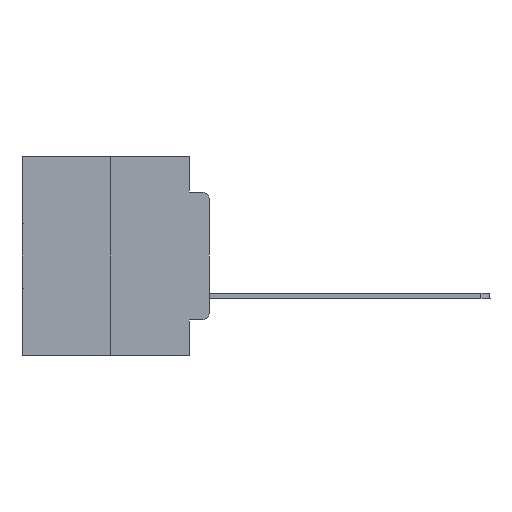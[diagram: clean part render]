
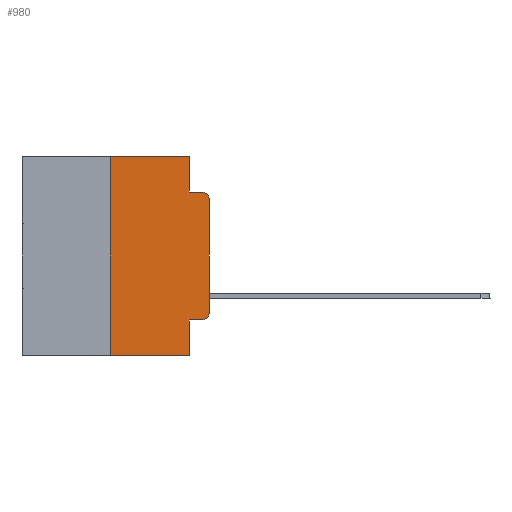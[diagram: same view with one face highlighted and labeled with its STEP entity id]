
A CAD part, left-side view. The second image highlights one B-rep face of the part: STEP entity #980.
In plain terms, the highlighted planar face has unit normal (-1, 0, 0).
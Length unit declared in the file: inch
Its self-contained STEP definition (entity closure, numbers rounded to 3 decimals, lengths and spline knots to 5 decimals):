
#5 = VECTOR ( 'NONE', #29559, 39.37008 ) ;
#486 = CARTESIAN_POINT ( 'NONE',  ( 0., 0., -0.3915 ) ) ;
#980 = ADVANCED_FACE ( 'NONE', ( #6678 ), #12092, .F. ) ;
#1792 = AXIS2_PLACEMENT_3D ( 'NONE', #6769, #27558, #7856 ) ;
#2124 = DIRECTION ( 'NONE',  ( 0., 0., -1. ) ) ;
#2141 = CARTESIAN_POINT ( 'NONE',  ( 0., 0.02, -0.1085 ) ) ;
#2211 = VERTEX_POINT ( 'NONE', #11360 ) ;
#2654 = VERTEX_POINT ( 'NONE', #27914 ) ;
#3202 = VERTEX_POINT ( 'NONE', #486 ) ;
#3818 = CARTESIAN_POINT ( 'NONE',  ( 0., 0.02, -0.0885 ) ) ;
#4131 = EDGE_CURVE ( 'NONE', #4163, #14780, #28726, .T. ) ;
#4163 = VERTEX_POINT ( 'NONE', #23117 ) ;
#4250 = EDGE_CURVE ( 'NONE', #11388, #4163, #6954, .T. ) ;
#4488 = DIRECTION ( 'NONE',  ( 0., -1., 0. ) ) ;
#4757 = VERTEX_POINT ( 'NONE', #7242 ) ;
#4994 = ORIENTED_EDGE ( 'NONE', *, *, #28750, .T. ) ;
#5087 = LINE ( 'NONE', #17276, #20365 ) ;
#5193 = ORIENTED_EDGE ( 'NONE', *, *, #13440, .F. ) ;
#5793 = EDGE_LOOP ( 'NONE', ( #4994, #28926, #23250, #27149, #14886, #5193, #23694, #9045, #26139, #23555 ) ) ;
#6230 = VERTEX_POINT ( 'NONE', #18127 ) ;
#6678 = FACE_OUTER_BOUND ( 'NONE', #5793, .T. ) ;
#6769 = CARTESIAN_POINT ( 'NONE',  ( 0., 0.02, -0.3915 ) ) ;
#6954 = LINE ( 'NONE', #18307, #26534 ) ;
#6980 = LINE ( 'NONE', #30104, #10633 ) ;
#7242 = CARTESIAN_POINT ( 'NONE',  ( 0., 0.02, -0.4115 ) ) ;
#7600 = DIRECTION ( 'NONE',  ( 1., 0., 0. ) ) ;
#7856 = DIRECTION ( 'NONE',  ( 0., 0., -1. ) ) ;
#7988 = LINE ( 'NONE', #10809, #5 ) ;
#8258 = EDGE_CURVE ( 'NONE', #4757, #3202, #11803, .T. ) ;
#9045 = ORIENTED_EDGE ( 'NONE', *, *, #11164, .F. ) ;
#10145 = DIRECTION ( 'NONE',  ( 0., 0., 1. ) ) ;
#10633 = VECTOR ( 'NONE', #22979, 39.37008 ) ;
#10809 = CARTESIAN_POINT ( 'NONE',  ( 0., 0.473, -0.5 ) ) ;
#10830 = CARTESIAN_POINT ( 'NONE',  ( 0., 0.25, 0. ) ) ;
#11164 = EDGE_CURVE ( 'NONE', #6230, #27643, #5087, .T. ) ;
#11336 = CIRCLE ( 'NONE', #18917, 0.02 ) ;
#11360 = CARTESIAN_POINT ( 'NONE',  ( 0., 0., -0.1085 ) ) ;
#11376 = DIRECTION ( 'NONE',  ( -1., 0., 0. ) ) ;
#11388 = VERTEX_POINT ( 'NONE', #22035 ) ;
#11675 = CARTESIAN_POINT ( 'NONE',  ( 0., 0.473, 0. ) ) ;
#11803 = CIRCLE ( 'NONE', #1792, 0.02 ) ;
#12092 = PLANE ( 'NONE',  #18562 ) ;
#12635 = EDGE_CURVE ( 'NONE', #6230, #4757, #17356, .T. ) ;
#12959 = DIRECTION ( 'NONE',  ( 0., -1., 0. ) ) ;
#13440 = EDGE_CURVE ( 'NONE', #2654, #28687, #27146, .T. ) ;
#14780 = VERTEX_POINT ( 'NONE', #3818 ) ;
#14886 = ORIENTED_EDGE ( 'NONE', *, *, #25388, .F. ) ;
#15371 = VECTOR ( 'NONE', #27470, 39.37008 ) ;
#15845 = CARTESIAN_POINT ( 'NONE',  ( 0., 0.051, -0.5 ) ) ;
#15999 = VECTOR ( 'NONE', #4488, 39.37008 ) ;
#16795 = CARTESIAN_POINT ( 'NONE',  ( 0., 0.473, 0. ) ) ;
#17162 = LINE ( 'NONE', #11675, #15371 ) ;
#17204 = CARTESIAN_POINT ( 'NONE',  ( 0., 0.25, 0. ) ) ;
#17276 = CARTESIAN_POINT ( 'NONE',  ( 0., 0.051, 0. ) ) ;
#17356 = LINE ( 'NONE', #27159, #22090 ) ;
#18127 = CARTESIAN_POINT ( 'NONE',  ( 0., 0.051, -0.4115 ) ) ;
#18307 = CARTESIAN_POINT ( 'NONE',  ( 0., 0.051, 0. ) ) ;
#18562 = AXIS2_PLACEMENT_3D ( 'NONE', #16795, #7600, #23817 ) ;
#18917 = AXIS2_PLACEMENT_3D ( 'NONE', #2141, #11376, #27559 ) ;
#19114 = DIRECTION ( 'NONE',  ( 0., 0., -1. ) ) ;
#20365 = VECTOR ( 'NONE', #19114, 39.37008 ) ;
#21574 = EDGE_CURVE ( 'NONE', #2211, #14780, #11336, .T. ) ;
#22035 = CARTESIAN_POINT ( 'NONE',  ( 0., 0.051, 0. ) ) ;
#22090 = VECTOR ( 'NONE', #12959, 39.37008 ) ;
#22979 = DIRECTION ( 'NONE',  ( 0., 0., 1. ) ) ;
#23117 = CARTESIAN_POINT ( 'NONE',  ( 0., 0.051, -0.0885 ) ) ;
#23250 = ORIENTED_EDGE ( 'NONE', *, *, #4131, .F. ) ;
#23555 = ORIENTED_EDGE ( 'NONE', *, *, #8258, .T. ) ;
#23694 = ORIENTED_EDGE ( 'NONE', *, *, #29824, .T. ) ;
#23817 = DIRECTION ( 'NONE',  ( 0., 0., -1. ) ) ;
#24615 = VECTOR ( 'NONE', #10145, 39.37008 ) ;
#25174 = CARTESIAN_POINT ( 'NONE',  ( 0., 0.051, -0.0885 ) ) ;
#25388 = EDGE_CURVE ( 'NONE', #28687, #11388, #17162, .T. ) ;
#26139 = ORIENTED_EDGE ( 'NONE', *, *, #12635, .T. ) ;
#26534 = VECTOR ( 'NONE', #2124, 39.37008 ) ;
#27146 = LINE ( 'NONE', #17204, #24615 ) ;
#27149 = ORIENTED_EDGE ( 'NONE', *, *, #4250, .F. ) ;
#27159 = CARTESIAN_POINT ( 'NONE',  ( 0., 0.051, -0.4115 ) ) ;
#27470 = DIRECTION ( 'NONE',  ( 0., -1., 0. ) ) ;
#27558 = DIRECTION ( 'NONE',  ( -1., 0., 0. ) ) ;
#27559 = DIRECTION ( 'NONE',  ( 0., 0., -1. ) ) ;
#27643 = VERTEX_POINT ( 'NONE', #15845 ) ;
#27914 = CARTESIAN_POINT ( 'NONE',  ( 0., 0.25, -0.5 ) ) ;
#28687 = VERTEX_POINT ( 'NONE', #10830 ) ;
#28726 = LINE ( 'NONE', #25174, #15999 ) ;
#28750 = EDGE_CURVE ( 'NONE', #3202, #2211, #6980, .T. ) ;
#28926 = ORIENTED_EDGE ( 'NONE', *, *, #21574, .T. ) ;
#29559 = DIRECTION ( 'NONE',  ( 0., -1., 0. ) ) ;
#29824 = EDGE_CURVE ( 'NONE', #2654, #27643, #7988, .T. ) ;
#30104 = CARTESIAN_POINT ( 'NONE',  ( 0., 0., 0. ) ) ;
